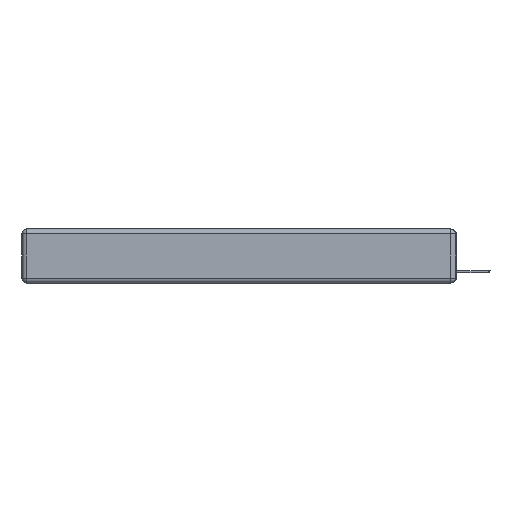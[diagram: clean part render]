
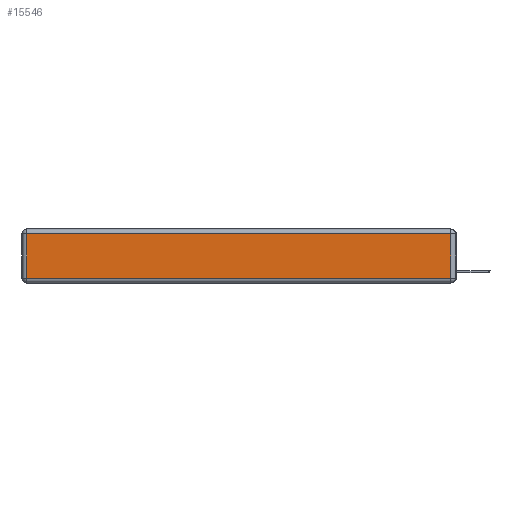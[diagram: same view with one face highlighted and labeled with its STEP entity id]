
A CAD part, left-side view. The second image highlights one B-rep face of the part: STEP entity #15546.
In plain terms, the highlighted planar face has unit normal (-1, 0, 0).
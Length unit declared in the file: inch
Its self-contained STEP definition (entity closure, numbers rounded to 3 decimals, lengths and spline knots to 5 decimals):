
#60 = ORIENTED_EDGE ( 'NONE', *, *, #2518, .T. ) ;
#254 = VERTEX_POINT ( 'NONE', #6204 ) ;
#2367 = AXIS2_PLACEMENT_3D ( 'NONE', #2586, #4293, #7359 ) ;
#2518 = EDGE_CURVE ( 'NONE', #8592, #10469, #10669, .T. ) ;
#2586 = CARTESIAN_POINT ( 'NONE',  ( 0., 0., -0.343 ) ) ;
#3930 = VERTEX_POINT ( 'NONE', #8021 ) ;
#4070 = ORIENTED_EDGE ( 'NONE', *, *, #14823, .T. ) ;
#4293 = DIRECTION ( 'NONE',  ( -1., 0., 0. ) ) ;
#4441 = VECTOR ( 'NONE', #9004, 39.37008 ) ;
#6204 = CARTESIAN_POINT ( 'NONE',  ( 0., 2.72, -0.313 ) ) ;
#7359 = DIRECTION ( 'NONE',  ( 0., 0., 1. ) ) ;
#7424 = VECTOR ( 'NONE', #18112, 39.37008 ) ;
#7665 = FACE_OUTER_BOUND ( 'NONE', #13063, .T. ) ;
#8021 = CARTESIAN_POINT ( 'NONE',  ( 0., 2.72, -0.03 ) ) ;
#8592 = VERTEX_POINT ( 'NONE', #16221 ) ;
#8599 = CARTESIAN_POINT ( 'NONE',  ( 0., 0.03, -0.343 ) ) ;
#9004 = DIRECTION ( 'NONE',  ( 0., -1., 0. ) ) ;
#9182 = PLANE ( 'NONE',  #2367 ) ;
#10469 = VERTEX_POINT ( 'NONE', #13185 ) ;
#10669 = LINE ( 'NONE', #8599, #15998 ) ;
#11479 = EDGE_CURVE ( 'NONE', #3930, #254, #14590, .T. ) ;
#11669 = EDGE_CURVE ( 'NONE', #10469, #3930, #11793, .T. ) ;
#11793 = LINE ( 'NONE', #12045, #18910 ) ;
#12035 = ORIENTED_EDGE ( 'NONE', *, *, #11479, .T. ) ;
#12045 = CARTESIAN_POINT ( 'NONE',  ( 0., 2.75, -0.03 ) ) ;
#13063 = EDGE_LOOP ( 'NONE', ( #4070, #60, #20206, #12035 ) ) ;
#13185 = CARTESIAN_POINT ( 'NONE',  ( 0., 0.03, -0.03 ) ) ;
#13725 = DIRECTION ( 'NONE',  ( 0., 1., 0. ) ) ;
#14590 = LINE ( 'NONE', #15023, #7424 ) ;
#14823 = EDGE_CURVE ( 'NONE', #254, #8592, #18257, .T. ) ;
#15023 = CARTESIAN_POINT ( 'NONE',  ( 0., 2.72, -0.343 ) ) ;
#15546 = ADVANCED_FACE ( 'NONE', ( #7665 ), #9182, .T. ) ;
#15998 = VECTOR ( 'NONE', #16691, 39.37008 ) ;
#16221 = CARTESIAN_POINT ( 'NONE',  ( 0., 0.03, -0.313 ) ) ;
#16691 = DIRECTION ( 'NONE',  ( 0., 0., 1. ) ) ;
#18112 = DIRECTION ( 'NONE',  ( 0., 0., -1. ) ) ;
#18257 = LINE ( 'NONE', #18760, #4441 ) ;
#18760 = CARTESIAN_POINT ( 'NONE',  ( 0., 0., -0.313 ) ) ;
#18910 = VECTOR ( 'NONE', #13725, 39.37008 ) ;
#20206 = ORIENTED_EDGE ( 'NONE', *, *, #11669, .T. ) ;
